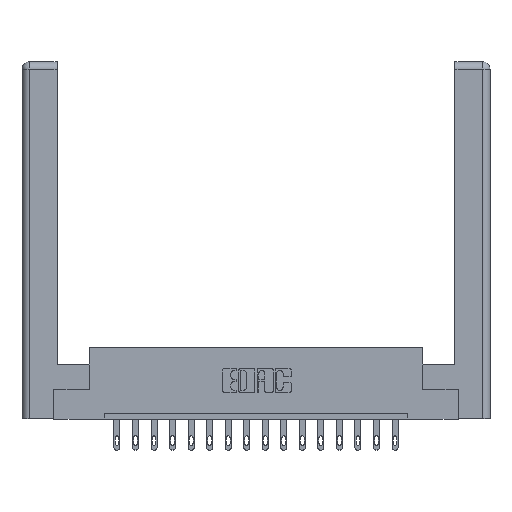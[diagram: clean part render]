
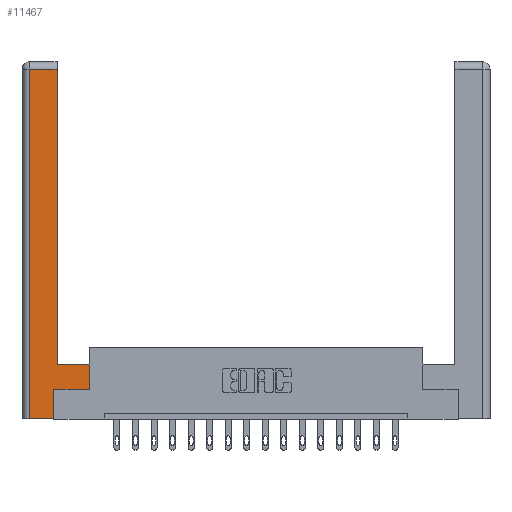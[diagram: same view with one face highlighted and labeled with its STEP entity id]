
A CAD part, top view. The second image highlights one B-rep face of the part: STEP entity #11467.
In plain terms, the highlighted planar face has unit normal (0, 0, 1).
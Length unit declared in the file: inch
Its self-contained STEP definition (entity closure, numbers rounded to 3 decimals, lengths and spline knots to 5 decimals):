
#498 = CARTESIAN_POINT ( 'NONE',  ( 0.0615, 2.94, 0. ) ) ;
#832 = CARTESIAN_POINT ( 'NONE',  ( 0., 0., 0. ) ) ;
#1533 = VECTOR ( 'NONE', #16088, 39.37008 ) ;
#1562 = VECTOR ( 'NONE', #3798, 39.37008 ) ;
#1782 = CARTESIAN_POINT ( 'NONE',  ( 0.265, 0.245, 0. ) ) ;
#2009 = VECTOR ( 'NONE', #2389, 39.37008 ) ;
#2195 = VECTOR ( 'NONE', #17393, 39.37008 ) ;
#2332 = LINE ( 'NONE', #17416, #9182 ) ;
#2389 = DIRECTION ( 'NONE',  ( 1., 0., 0. ) ) ;
#2423 = ORIENTED_EDGE ( 'NONE', *, *, #8679, .T. ) ;
#2469 = CARTESIAN_POINT ( 'NONE',  ( 0.265, 0., 0. ) ) ;
#2635 = DIRECTION ( 'NONE',  ( -1., 0., 0. ) ) ;
#2827 = EDGE_CURVE ( 'NONE', #13556, #14543, #12745, .T. ) ;
#2973 = ORIENTED_EDGE ( 'NONE', *, *, #8946, .T. ) ;
#3083 = LINE ( 'NONE', #7944, #2195 ) ;
#3443 = LINE ( 'NONE', #7223, #11996 ) ;
#3798 = DIRECTION ( 'NONE',  ( 0., 1., 0. ) ) ;
#4201 = CARTESIAN_POINT ( 'NONE',  ( 0.0615, 0., 0. ) ) ;
#4744 = VERTEX_POINT ( 'NONE', #7817 ) ;
#4814 = LINE ( 'NONE', #5385, #2009 ) ;
#4959 = DIRECTION ( 'NONE',  ( 0., 0., -1. ) ) ;
#5206 = LINE ( 'NONE', #10564, #1533 ) ;
#5259 = CARTESIAN_POINT ( 'NONE',  ( 0.0615, 2.94, 0. ) ) ;
#5262 = DIRECTION ( 'NONE',  ( 0., 1., 0. ) ) ;
#5385 = CARTESIAN_POINT ( 'NONE',  ( 0.265, 0., 0. ) ) ;
#5458 = VECTOR ( 'NONE', #2635, 39.37008 ) ;
#5858 = VECTOR ( 'NONE', #6585, 39.37008 ) ;
#6506 = EDGE_LOOP ( 'NONE', ( #15181, #12567, #2423, #16857, #8670, #2973, #13042, #7616 ) ) ;
#6538 = EDGE_CURVE ( 'NONE', #8059, #17657, #2332, .T. ) ;
#6585 = DIRECTION ( 'NONE',  ( 0., -1., 0. ) ) ;
#7223 = CARTESIAN_POINT ( 'NONE',  ( 0.295, 0.45, 0. ) ) ;
#7616 = ORIENTED_EDGE ( 'NONE', *, *, #16968, .T. ) ;
#7817 = CARTESIAN_POINT ( 'NONE',  ( 0.565, 0.245, 0. ) ) ;
#7818 = LINE ( 'NONE', #9354, #1562 ) ;
#7846 = CARTESIAN_POINT ( 'NONE',  ( 0.295, 2.94, 0. ) ) ;
#7944 = CARTESIAN_POINT ( 'NONE',  ( 0.565, 0.45, 0. ) ) ;
#7984 = AXIS2_PLACEMENT_3D ( 'NONE', #832, #4959, #14453 ) ;
#8059 = VERTEX_POINT ( 'NONE', #2469 ) ;
#8124 = VERTEX_POINT ( 'NONE', #4201 ) ;
#8486 = EDGE_CURVE ( 'NONE', #4744, #15499, #3083, .T. ) ;
#8670 = ORIENTED_EDGE ( 'NONE', *, *, #6538, .T. ) ;
#8679 = EDGE_CURVE ( 'NONE', #14543, #8124, #16786, .T. ) ;
#8946 = EDGE_CURVE ( 'NONE', #17657, #4744, #5206, .T. ) ;
#9182 = VECTOR ( 'NONE', #5262, 39.37008 ) ;
#9354 = CARTESIAN_POINT ( 'NONE',  ( 0.295, 3., 0. ) ) ;
#10564 = CARTESIAN_POINT ( 'NONE',  ( 0.565, 0.245, 0. ) ) ;
#11467 = ADVANCED_FACE ( 'NONE', ( #13084 ), #12706, .F. ) ;
#11996 = VECTOR ( 'NONE', #14064, 39.37008 ) ;
#12135 = VERTEX_POINT ( 'NONE', #16772 ) ;
#12144 = CARTESIAN_POINT ( 'NONE',  ( 0.0615, 0., 0. ) ) ;
#12567 = ORIENTED_EDGE ( 'NONE', *, *, #2827, .T. ) ;
#12706 = PLANE ( 'NONE',  #7984 ) ;
#12745 = LINE ( 'NONE', #5259, #5458 ) ;
#13042 = ORIENTED_EDGE ( 'NONE', *, *, #8486, .T. ) ;
#13084 = FACE_OUTER_BOUND ( 'NONE', #6506, .T. ) ;
#13453 = CARTESIAN_POINT ( 'NONE',  ( 0.565, 0.45, 0. ) ) ;
#13556 = VERTEX_POINT ( 'NONE', #7846 ) ;
#14064 = DIRECTION ( 'NONE',  ( -1., 0., 0. ) ) ;
#14453 = DIRECTION ( 'NONE',  ( -1., 0., 0. ) ) ;
#14543 = VERTEX_POINT ( 'NONE', #498 ) ;
#15131 = EDGE_CURVE ( 'NONE', #8124, #8059, #4814, .T. ) ;
#15181 = ORIENTED_EDGE ( 'NONE', *, *, #15383, .T. ) ;
#15383 = EDGE_CURVE ( 'NONE', #12135, #13556, #7818, .T. ) ;
#15499 = VERTEX_POINT ( 'NONE', #13453 ) ;
#16088 = DIRECTION ( 'NONE',  ( 1., 0., 0. ) ) ;
#16772 = CARTESIAN_POINT ( 'NONE',  ( 0.295, 0.45, 0. ) ) ;
#16786 = LINE ( 'NONE', #12144, #5858 ) ;
#16857 = ORIENTED_EDGE ( 'NONE', *, *, #15131, .T. ) ;
#16968 = EDGE_CURVE ( 'NONE', #15499, #12135, #3443, .T. ) ;
#17393 = DIRECTION ( 'NONE',  ( 0., 1., 0. ) ) ;
#17416 = CARTESIAN_POINT ( 'NONE',  ( 0.265, 0.245, 0. ) ) ;
#17657 = VERTEX_POINT ( 'NONE', #1782 ) ;
